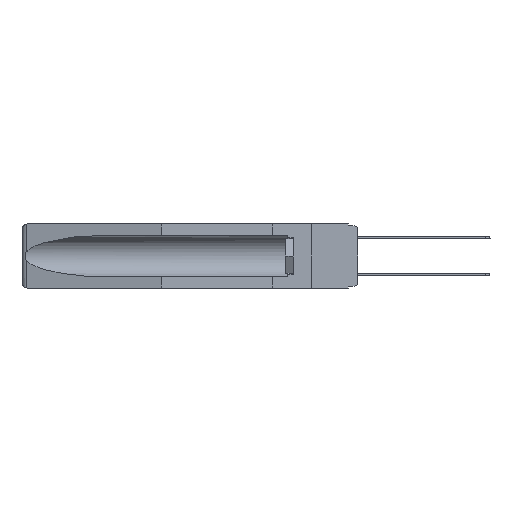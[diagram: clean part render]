
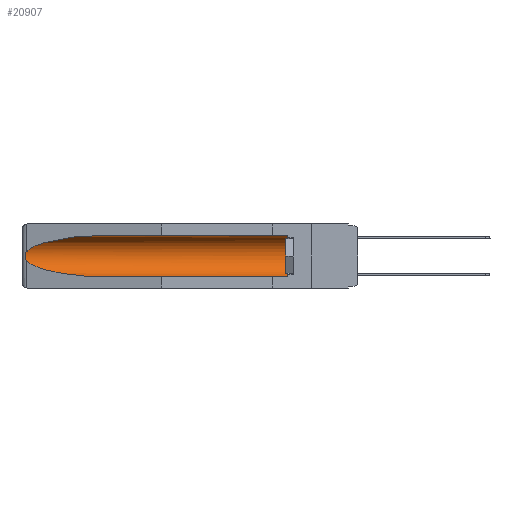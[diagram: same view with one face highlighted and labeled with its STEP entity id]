
A CAD part, left-side view. The second image highlights one B-rep face of the part: STEP entity #20907.
In plain terms, the highlighted cylindrical face has radius 2.857 mm (diameter 5.715 mm), a partial arc.
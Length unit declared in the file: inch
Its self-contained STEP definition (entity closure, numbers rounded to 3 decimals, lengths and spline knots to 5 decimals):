
#439 = CARTESIAN_POINT ( 'NONE',  ( 0.26537, 1.52718, -0.19328 ) ) ;
#557 = CARTESIAN_POINT ( 'NONE',  ( 0.155, 1.07973, -0.284 ) ) ;
#778 = CARTESIAN_POINT ( 'NONE',  ( 0.155, -0.30754, -0.1715 ) ) ;
#810 = CARTESIAN_POINT ( 'NONE',  ( 0.2675, 1.53308, -0.17534 ) ) ;
#1281 = CIRCLE ( 'NONE', #21202, 0.1125 ) ;
#2504 = ORIENTED_EDGE ( 'NONE', *, *, #21798, .T. ) ;
#3021 = VERTEX_POINT ( 'NONE', #14929 ) ;
#3931 = CARTESIAN_POINT ( 'NONE',  ( 0.155, 1.07973, -0.059 ) ) ;
#4263 = DIRECTION ( 'NONE',  ( 0., 1., 0. ) ) ;
#4397 = CARTESIAN_POINT ( 'NONE',  ( 0.155, -0.30754, -0.059 ) ) ;
#4711 = CYLINDRICAL_SURFACE ( 'NONE', #12359, 0.1125 ) ;
#4998 = ORIENTED_EDGE ( 'NONE', *, *, #13281, .T. ) ;
#6670 = CARTESIAN_POINT ( 'NONE',  ( 0.26655, 1.53094, -0.18657 ) ) ;
#7052 = CARTESIAN_POINT ( 'NONE',  ( 0.25451, 1.48313, -0.24835 ) ) ;
#7375 = VECTOR ( 'NONE', #12214, 39.37008 ) ;
#8002 = VECTOR ( 'NONE', #4263, 39.37008 ) ;
#8470 =( BOUNDED_CURVE ( )  B_SPLINE_CURVE ( 3, ( #3931, #13537, #9954, #17627 ),
 .UNSPECIFIED., .F., .F. ) 
 B_SPLINE_CURVE_WITH_KNOTS ( ( 4, 4 ),
 ( 4.71239, 6.08839 ),
 .UNSPECIFIED. ) 
 CURVE ( )  GEOMETRIC_REPRESENTATION_ITEM ( )  RATIONAL_B_SPLINE_CURVE ( ( 1., 0.848, 0.848, 1. ) ) 
 REPRESENTATION_ITEM ( '' )  );
#8714 = CARTESIAN_POINT ( 'NONE',  ( 0.26537, 1.52718, -0.14972 ) ) ;
#9257 = CARTESIAN_POINT ( 'NONE',  ( 0.26537, 1.52718, -0.14972 ) ) ;
#9897 = EDGE_CURVE ( 'NONE', #3021, #16052, #8470, .T. ) ;
#9954 = CARTESIAN_POINT ( 'NONE',  ( 0.25451, 1.48313, -0.09465 ) ) ;
#10265 = CARTESIAN_POINT ( 'NONE',  ( 0.2675, 1.53308, -0.16763 ) ) ;
#10348 = FACE_OUTER_BOUND ( 'NONE', #22184, .T. ) ;
#10508 = CARTESIAN_POINT ( 'NONE',  ( 0.26537, 1.52718, -0.19328 ) ) ;
#10606 = DIRECTION ( 'NONE',  ( 0., 1., 0. ) ) ;
#11032 = VERTEX_POINT ( 'NONE', #15834 ) ;
#11687 = ORIENTED_EDGE ( 'NONE', *, *, #9897, .T. ) ;
#12186 = CARTESIAN_POINT ( 'NONE',  ( 0.26654, 1.53092, -0.15636 ) ) ;
#12214 = DIRECTION ( 'NONE',  ( 0., 1., 0. ) ) ;
#12309 = ORIENTED_EDGE ( 'NONE', *, *, #24597, .F. ) ;
#12359 = AXIS2_PLACEMENT_3D ( 'NONE', #778, #10606, #18140 ) ;
#12426 = CARTESIAN_POINT ( 'NONE',  ( 0.26597, 1.52961, -0.15275 ) ) ;
#12626 = VERTEX_POINT ( 'NONE', #20443 ) ;
#13281 = EDGE_CURVE ( 'NONE', #16052, #12626, #24349, .T. ) ;
#13537 = CARTESIAN_POINT ( 'NONE',  ( 0.21114, 1.30732, -0.059 ) ) ;
#13993 = CARTESIAN_POINT ( 'NONE',  ( 0.155, -0.30754, -0.284 ) ) ;
#14692 =( BOUNDED_CURVE ( )  B_SPLINE_CURVE ( 3, ( #10508, #7052, #20345, #24423 ),
 .UNSPECIFIED., .F., .F. ) 
 B_SPLINE_CURVE_WITH_KNOTS ( ( 4, 4 ),
 ( 0.1948, 1.5708 ),
 .UNSPECIFIED. ) 
 CURVE ( )  GEOMETRIC_REPRESENTATION_ITEM ( )  RATIONAL_B_SPLINE_CURVE ( ( 1., 0.848, 0.848, 1. ) ) 
 REPRESENTATION_ITEM ( '' )  );
#14929 = CARTESIAN_POINT ( 'NONE',  ( 0.155, 1.07973, -0.059 ) ) ;
#15834 = CARTESIAN_POINT ( 'NONE',  ( 0.155, 0.126, -0.059 ) ) ;
#15917 = LINE ( 'NONE', #13993, #8002 ) ;
#16052 = VERTEX_POINT ( 'NONE', #9257 ) ;
#16399 = CARTESIAN_POINT ( 'NONE',  ( 0.2673, 1.5327, -0.16383 ) ) ;
#16844 = CARTESIAN_POINT ( 'NONE',  ( 0.155, 0.126, -0.1715 ) ) ;
#16960 = DIRECTION ( 'NONE',  ( 0., 0., 1. ) ) ;
#17627 = CARTESIAN_POINT ( 'NONE',  ( 0.26537, 1.52718, -0.14972 ) ) ;
#18140 = DIRECTION ( 'NONE',  ( 0., 0., 1. ) ) ;
#18630 = EDGE_CURVE ( 'NONE', #25062, #11032, #1281, .T. ) ;
#19953 = EDGE_CURVE ( 'NONE', #11032, #3021, #21898, .T. ) ;
#20060 = CARTESIAN_POINT ( 'NONE',  ( 0.155, 0.126, -0.284 ) ) ;
#20210 = CARTESIAN_POINT ( 'NONE',  ( 0.2673, 1.53269, -0.17917 ) ) ;
#20345 = CARTESIAN_POINT ( 'NONE',  ( 0.21114, 1.30732, -0.284 ) ) ;
#20443 = CARTESIAN_POINT ( 'NONE',  ( 0.26537, 1.52718, -0.19328 ) ) ;
#20581 = ORIENTED_EDGE ( 'NONE', *, *, #18630, .T. ) ;
#20907 = ADVANCED_FACE ( 'NONE', ( #10348 ), #4711, .F. ) ;
#21202 = AXIS2_PLACEMENT_3D ( 'NONE', #16844, #24862, #16960 ) ;
#21670 = VERTEX_POINT ( 'NONE', #557 ) ;
#21798 = EDGE_CURVE ( 'NONE', #12626, #21670, #14692, .T. ) ;
#21898 = LINE ( 'NONE', #4397, #7375 ) ;
#22184 = EDGE_LOOP ( 'NONE', ( #11687, #4998, #2504, #12309, #20581, #23313 ) ) ;
#22244 = CARTESIAN_POINT ( 'NONE',  ( 0.26597, 1.5296, -0.19026 ) ) ;
#23313 = ORIENTED_EDGE ( 'NONE', *, *, #19953, .T. ) ;
#24349 = B_SPLINE_CURVE_WITH_KNOTS ( 'NONE', 3,
 ( #8714, #12426, #12186, #16399, #10265, #810, #20210, #6670, #22244, #439 ),
 .UNSPECIFIED., .F., .F.,
 ( 4, 2, 2, 2, 4 ),
 ( 0., 0.00029, 0.00058, 0.00087, 0.00117 ),
 .UNSPECIFIED. ) ;
#24423 = CARTESIAN_POINT ( 'NONE',  ( 0.155, 1.07973, -0.284 ) ) ;
#24597 = EDGE_CURVE ( 'NONE', #25062, #21670, #15917, .T. ) ;
#24862 = DIRECTION ( 'NONE',  ( 0., -1., 0. ) ) ;
#25062 = VERTEX_POINT ( 'NONE', #20060 ) ;
